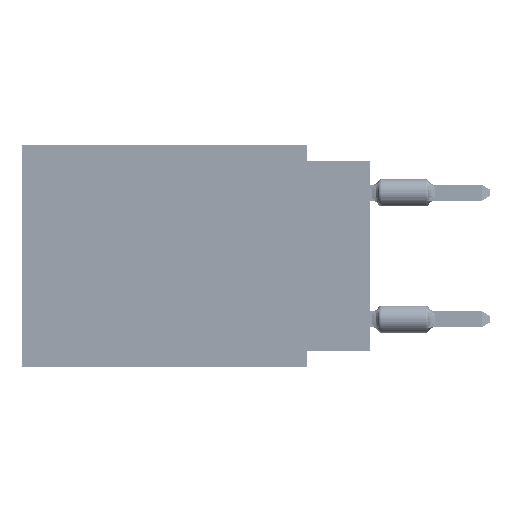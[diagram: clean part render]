
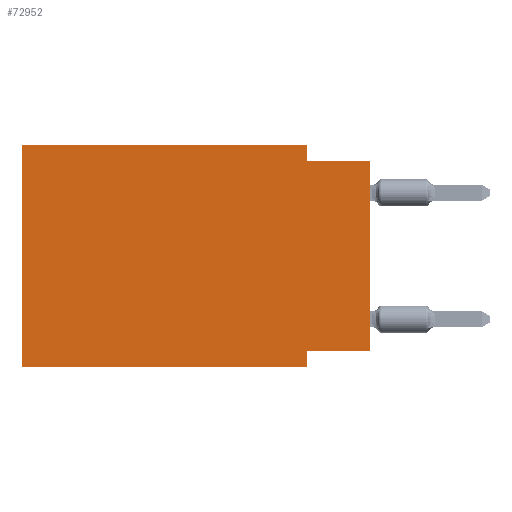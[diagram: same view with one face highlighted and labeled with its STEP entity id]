
A CAD part, left-side view. The second image highlights one B-rep face of the part: STEP entity #72952.
In plain terms, the highlighted planar face has unit normal (-1, 0, 0).
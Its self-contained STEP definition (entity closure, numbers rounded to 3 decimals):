
#355 = EDGE_CURVE ( 'NONE', #20500, #58291, #73226, .T. ) ;
#2498 = CARTESIAN_POINT ( 'NONE',  ( 0., 13.97, -8.89 ) ) ;
#2660 = DIRECTION ( 'NONE',  ( 0., 0., 1. ) ) ;
#3517 = DIRECTION ( 'NONE',  ( 0., 0., 1. ) ) ;
#4665 = EDGE_CURVE ( 'NONE', #55528, #84548, #86200, .T. ) ;
#5242 = CARTESIAN_POINT ( 'NONE',  ( 0., 2.54, -8.255 ) ) ;
#11095 = CARTESIAN_POINT ( 'NONE',  ( 0., 13.97, 0. ) ) ;
#12167 = DIRECTION ( 'NONE',  ( 0., 1., 0. ) ) ;
#13443 = CARTESIAN_POINT ( 'NONE',  ( 0., 0., -0.635 ) ) ;
#14261 = EDGE_LOOP ( 'NONE', ( #20838, #79146, #22691, #32128, #26383, #37159, #67108, #45565 ) ) ;
#15704 = CARTESIAN_POINT ( 'NONE',  ( 0., 2.54, -8.89 ) ) ;
#20500 = VERTEX_POINT ( 'NONE', #57724 ) ;
#20759 = LINE ( 'NONE', #92747, #31160 ) ;
#20838 = ORIENTED_EDGE ( 'NONE', *, *, #54599, .T. ) ;
#22039 = DIRECTION ( 'NONE',  ( 0., -1., 0. ) ) ;
#22691 = ORIENTED_EDGE ( 'NONE', *, *, #59724, .F. ) ;
#24249 = VECTOR ( 'NONE', #3517, 1000. ) ;
#26383 = ORIENTED_EDGE ( 'NONE', *, *, #57998, .F. ) ;
#28461 = CARTESIAN_POINT ( 'NONE',  ( 0., 0., -0.635 ) ) ;
#31160 = VECTOR ( 'NONE', #55818, 1000. ) ;
#31302 = CARTESIAN_POINT ( 'NONE',  ( 0., 0., -8.255 ) ) ;
#32128 = ORIENTED_EDGE ( 'NONE', *, *, #39694, .F. ) ;
#34343 = CARTESIAN_POINT ( 'NONE',  ( 0., 0., -8.255 ) ) ;
#34560 = CARTESIAN_POINT ( 'NONE',  ( 0., 2.54, -8.89 ) ) ;
#36036 = DIRECTION ( 'NONE',  ( 0., 0., -1. ) ) ;
#37159 = ORIENTED_EDGE ( 'NONE', *, *, #47711, .T. ) ;
#37267 = LINE ( 'NONE', #96773, #54289 ) ;
#38013 = DIRECTION ( 'NONE',  ( 0., -1., 0. ) ) ;
#39352 = VECTOR ( 'NONE', #38013, 1000. ) ;
#39694 = EDGE_CURVE ( 'NONE', #41345, #53125, #37267, .T. ) ;
#40079 = CARTESIAN_POINT ( 'NONE',  ( 0., 13.97, 0. ) ) ;
#40462 = CARTESIAN_POINT ( 'NONE',  ( 0., 0., 0. ) ) ;
#41345 = VERTEX_POINT ( 'NONE', #11095 ) ;
#42880 = VECTOR ( 'NONE', #22039, 1000. ) ;
#45565 = ORIENTED_EDGE ( 'NONE', *, *, #60496, .F. ) ;
#47340 = AXIS2_PLACEMENT_3D ( 'NONE', #66030, #97005, #36036 ) ;
#47463 = LINE ( 'NONE', #40079, #93812 ) ;
#47711 = EDGE_CURVE ( 'NONE', #97216, #84548, #54698, .T. ) ;
#52702 = FACE_OUTER_BOUND ( 'NONE', #14261, .T. ) ;
#52738 = VERTEX_POINT ( 'NONE', #31302 ) ;
#53125 = VERTEX_POINT ( 'NONE', #75483 ) ;
#54289 = VECTOR ( 'NONE', #58435, 1000. ) ;
#54599 = EDGE_CURVE ( 'NONE', #52738, #58291, #56200, .T. ) ;
#54698 = LINE ( 'NONE', #2498, #39352 ) ;
#55528 = VERTEX_POINT ( 'NONE', #5242 ) ;
#55818 = DIRECTION ( 'NONE',  ( 0., 0., -1. ) ) ;
#56200 = LINE ( 'NONE', #40462, #24249 ) ;
#56954 = LINE ( 'NONE', #34343, #75357 ) ;
#57356 = CARTESIAN_POINT ( 'NONE',  ( 0., 13.97, -8.89 ) ) ;
#57724 = CARTESIAN_POINT ( 'NONE',  ( 0., 2.54, -0.635 ) ) ;
#57998 = EDGE_CURVE ( 'NONE', #97216, #41345, #47463, .T. ) ;
#58291 = VERTEX_POINT ( 'NONE', #13443 ) ;
#58435 = DIRECTION ( 'NONE',  ( 0., -1., 0. ) ) ;
#59724 = EDGE_CURVE ( 'NONE', #53125, #20500, #20759, .T. ) ;
#60496 = EDGE_CURVE ( 'NONE', #52738, #55528, #56954, .T. ) ;
#66030 = CARTESIAN_POINT ( 'NONE',  ( 0., 13.97, 0. ) ) ;
#67108 = ORIENTED_EDGE ( 'NONE', *, *, #4665, .F. ) ;
#72952 = ADVANCED_FACE ( 'NONE', ( #52702 ), #81766, .F. ) ;
#73226 = LINE ( 'NONE', #28461, #42880 ) ;
#75357 = VECTOR ( 'NONE', #12167, 1000. ) ;
#75483 = CARTESIAN_POINT ( 'NONE',  ( 0., 2.54, 0. ) ) ;
#78818 = DIRECTION ( 'NONE',  ( 0., 0., -1. ) ) ;
#79146 = ORIENTED_EDGE ( 'NONE', *, *, #355, .F. ) ;
#81766 = PLANE ( 'NONE',  #47340 ) ;
#84548 = VERTEX_POINT ( 'NONE', #15704 ) ;
#85597 = VECTOR ( 'NONE', #78818, 1000. ) ;
#86200 = LINE ( 'NONE', #34560, #85597 ) ;
#92747 = CARTESIAN_POINT ( 'NONE',  ( 0., 2.54, 0. ) ) ;
#93812 = VECTOR ( 'NONE', #2660, 1000. ) ;
#96773 = CARTESIAN_POINT ( 'NONE',  ( 0., 13.97, 0. ) ) ;
#97005 = DIRECTION ( 'NONE',  ( 1., 0., 0. ) ) ;
#97216 = VERTEX_POINT ( 'NONE', #57356 ) ;
